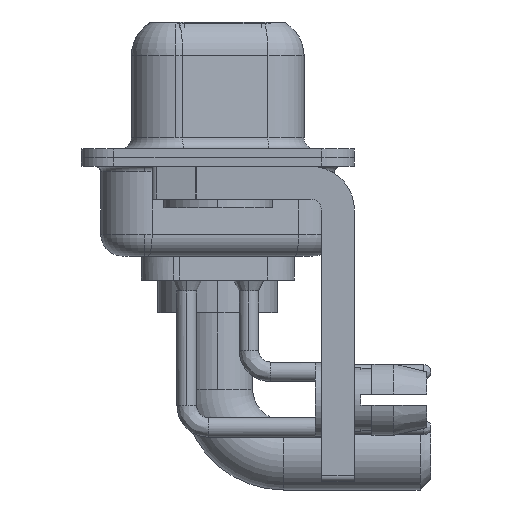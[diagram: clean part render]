
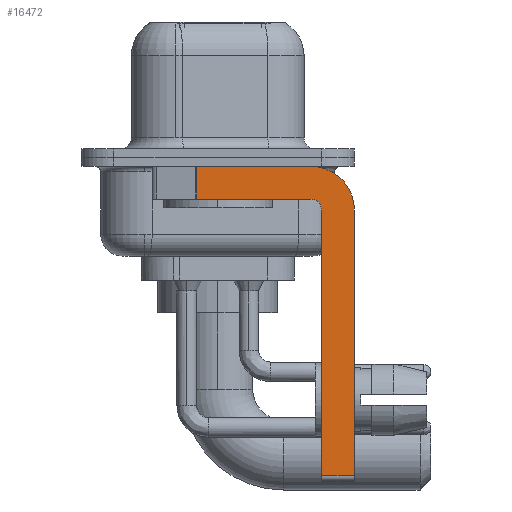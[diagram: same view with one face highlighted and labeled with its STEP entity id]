
A CAD part, left-side view. The second image highlights one B-rep face of the part: STEP entity #16472.
In plain terms, the highlighted planar face has unit normal (-1, 0, 0).
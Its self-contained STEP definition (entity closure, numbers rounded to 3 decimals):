
#4 = LINE ( 'NONE', #1574, #11320 ) ;
#31 = VERTEX_POINT ( 'NONE', #9047 ) ;
#304 = DIRECTION ( 'NONE',  ( 0., 0., -1. ) ) ;
#944 = CARTESIAN_POINT ( 'NONE',  ( -2.9, -6.25, -14.55 ) ) ;
#1298 = ORIENTED_EDGE ( 'NONE', *, *, #7771, .F. ) ;
#1574 = CARTESIAN_POINT ( 'NONE',  ( -2.9, 3., -0.4 ) ) ;
#1614 = AXIS2_PLACEMENT_3D ( 'NONE', #14747, #8193, #9571 ) ;
#2076 = DIRECTION ( 'NONE',  ( 0., -1., 0. ) ) ;
#2562 = VERTEX_POINT ( 'NONE', #9479 ) ;
#2605 = EDGE_CURVE ( 'NONE', #2861, #31, #4516, .T. ) ;
#2861 = VERTEX_POINT ( 'NONE', #4843 ) ;
#3266 = EDGE_CURVE ( 'NONE', #4846, #2562, #4, .T. ) ;
#4277 = VECTOR ( 'NONE', #12117, 1000. ) ;
#4516 = LINE ( 'NONE', #14018, #17702 ) ;
#4821 = DIRECTION ( 'NONE',  ( 0., -1., 0. ) ) ;
#4824 = ORIENTED_EDGE ( 'NONE', *, *, #12201, .F. ) ;
#4843 = CARTESIAN_POINT ( 'NONE',  ( -2.9, -4.75, -14.55 ) ) ;
#4846 = VERTEX_POINT ( 'NONE', #17349 ) ;
#5070 = CARTESIAN_POINT ( 'NONE',  ( -2.9, -4.25, -2.4 ) ) ;
#5153 = EDGE_CURVE ( 'NONE', #2861, #10025, #5420, .T. ) ;
#5324 = CARTESIAN_POINT ( 'NONE',  ( -2.9, -4.25, -1.9 ) ) ;
#5420 = LINE ( 'NONE', #10064, #10970 ) ;
#5665 = CARTESIAN_POINT ( 'NONE',  ( -2.9, -6.25, -2.4 ) ) ;
#5934 = CIRCLE ( 'NONE', #15379, 0.5 ) ;
#6693 = EDGE_CURVE ( 'NONE', #2562, #13500, #14009, .T. ) ;
#7771 = EDGE_CURVE ( 'NONE', #13500, #10025, #8926, .T. ) ;
#7914 = ORIENTED_EDGE ( 'NONE', *, *, #16325, .F. ) ;
#8193 = DIRECTION ( 'NONE',  ( 1., 0., 0. ) ) ;
#8253 = CARTESIAN_POINT ( 'NONE',  ( -2.9, -6.25, -2.4 ) ) ;
#8327 = DIRECTION ( 'NONE',  ( 1., 0., 0. ) ) ;
#8475 = LINE ( 'NONE', #13239, #12342 ) ;
#8926 = LINE ( 'NONE', #5665, #4277 ) ;
#9047 = CARTESIAN_POINT ( 'NONE',  ( -2.9, -4.75, -2.4 ) ) ;
#9479 = CARTESIAN_POINT ( 'NONE',  ( -2.9, -4.25, -0.4 ) ) ;
#9571 = DIRECTION ( 'NONE',  ( 0., 0., -1. ) ) ;
#9783 = VECTOR ( 'NONE', #19550, 1000. ) ;
#9789 = PLANE ( 'NONE',  #1614 ) ;
#9920 = VERTEX_POINT ( 'NONE', #14950 ) ;
#9937 = ORIENTED_EDGE ( 'NONE', *, *, #5153, .T. ) ;
#10025 = VERTEX_POINT ( 'NONE', #944 ) ;
#10064 = CARTESIAN_POINT ( 'NONE',  ( -2.9, -4.25, -14.55 ) ) ;
#10338 = DIRECTION ( 'NONE',  ( 0., 0., -1. ) ) ;
#10902 = ORIENTED_EDGE ( 'NONE', *, *, #2605, .F. ) ;
#10970 = VECTOR ( 'NONE', #2076, 1000. ) ;
#11267 = FACE_OUTER_BOUND ( 'NONE', #13263, .T. ) ;
#11320 = VECTOR ( 'NONE', #4821, 1000. ) ;
#11643 = VERTEX_POINT ( 'NONE', #5324 ) ;
#11676 = AXIS2_PLACEMENT_3D ( 'NONE', #5070, #8327, #10338 ) ;
#12117 = DIRECTION ( 'NONE',  ( 0., 0., -1. ) ) ;
#12152 = CARTESIAN_POINT ( 'NONE',  ( -2.9, -4.25, -2.4 ) ) ;
#12201 = EDGE_CURVE ( 'NONE', #11643, #9920, #17973, .T. ) ;
#12342 = VECTOR ( 'NONE', #304, 1000. ) ;
#13209 = ORIENTED_EDGE ( 'NONE', *, *, #6693, .F. ) ;
#13239 = CARTESIAN_POINT ( 'NONE',  ( -2.9, 0.978, -1.9 ) ) ;
#13263 = EDGE_LOOP ( 'NONE', ( #14803, #15998, #4824, #7914, #10902, #9937, #1298, #13209 ) ) ;
#13500 = VERTEX_POINT ( 'NONE', #8253 ) ;
#14009 = CIRCLE ( 'NONE', #11676, 2. ) ;
#14018 = CARTESIAN_POINT ( 'NONE',  ( -2.9, -4.75, -14.8 ) ) ;
#14747 = CARTESIAN_POINT ( 'NONE',  ( -2.9, -4.25, -2.4 ) ) ;
#14803 = ORIENTED_EDGE ( 'NONE', *, *, #3266, .F. ) ;
#14950 = CARTESIAN_POINT ( 'NONE',  ( -2.9, 0.978, -1.9 ) ) ;
#15379 = AXIS2_PLACEMENT_3D ( 'NONE', #12152, #18363, #16905 ) ;
#15764 = EDGE_CURVE ( 'NONE', #4846, #9920, #8475, .T. ) ;
#15998 = ORIENTED_EDGE ( 'NONE', *, *, #15764, .T. ) ;
#16325 = EDGE_CURVE ( 'NONE', #31, #11643, #5934, .T. ) ;
#16472 = ADVANCED_FACE ( 'NONE', ( #11267 ), #9789, .F. ) ;
#16905 = DIRECTION ( 'NONE',  ( 0., 0., 1. ) ) ;
#17293 = DIRECTION ( 'NONE',  ( 0., 0., 1. ) ) ;
#17349 = CARTESIAN_POINT ( 'NONE',  ( -2.9, 0.978, -0.4 ) ) ;
#17702 = VECTOR ( 'NONE', #17293, 1000. ) ;
#17973 = LINE ( 'NONE', #19231, #9783 ) ;
#18363 = DIRECTION ( 'NONE',  ( -1., 0., 0. ) ) ;
#19231 = CARTESIAN_POINT ( 'NONE',  ( -2.9, -4.25, -1.9 ) ) ;
#19550 = DIRECTION ( 'NONE',  ( 0., 1., 0. ) ) ;
